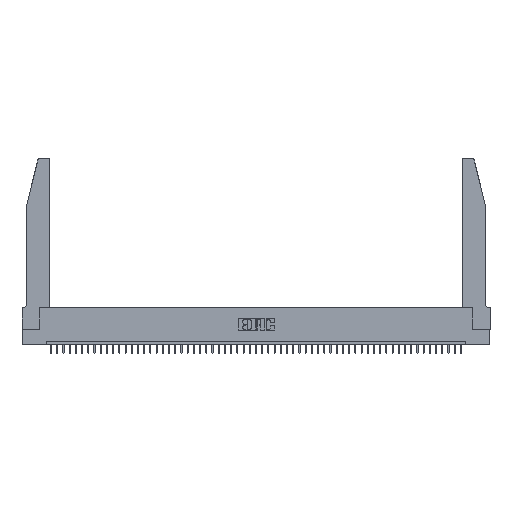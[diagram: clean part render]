
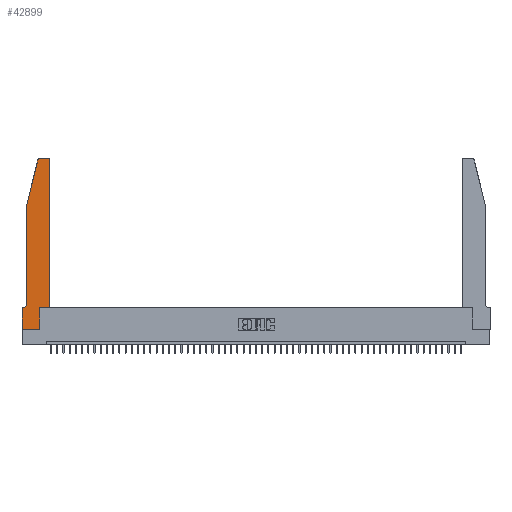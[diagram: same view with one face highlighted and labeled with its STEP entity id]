
A CAD part, top view. The second image highlights one B-rep face of the part: STEP entity #42899.
In plain terms, the highlighted planar face has unit normal (0, 0, 1).
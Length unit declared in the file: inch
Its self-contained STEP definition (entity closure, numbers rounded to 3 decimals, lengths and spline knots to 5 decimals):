
#58 = CARTESIAN_POINT ( 'NONE',  ( 0., 0., 0.37 ) ) ;
#282 = CARTESIAN_POINT ( 'NONE',  ( 0.0755, 2., 0.37 ) ) ;
#797 = LINE ( 'NONE', #282, #17827 ) ;
#1139 = VERTEX_POINT ( 'NONE', #1203 ) ;
#1203 = CARTESIAN_POINT ( 'NONE',  ( 0.4505, 2.72, 0.37 ) ) ;
#2063 = EDGE_CURVE ( 'NONE', #24006, #1139, #30928, .T. ) ;
#2872 = LINE ( 'NONE', #50670, #32849 ) ;
#2934 = CARTESIAN_POINT ( 'NONE',  ( 0.2865, 0.35, 0.37 ) ) ;
#3099 = CARTESIAN_POINT ( 'NONE',  ( 0.4505, 0.35, 0.37 ) ) ;
#3978 = LINE ( 'NONE', #7670, #49486 ) ;
#4060 = EDGE_CURVE ( 'NONE', #22851, #24006, #2872, .T. ) ;
#4466 = DIRECTION ( 'NONE',  ( 0., -1., 0. ) ) ;
#5199 = DIRECTION ( 'NONE',  ( 1., 0., 0. ) ) ;
#5670 = CIRCLE ( 'NONE', #44254, 0.03 ) ;
#5770 = CARTESIAN_POINT ( 'NONE',  ( 0., 0., 0.37 ) ) ;
#5868 = CARTESIAN_POINT ( 'NONE',  ( 0.25487, 2.72718, 0.37 ) ) ;
#6848 = LINE ( 'NONE', #15014, #40500 ) ;
#7275 = LINE ( 'NONE', #35645, #19015 ) ;
#7537 = CARTESIAN_POINT ( 'NONE',  ( 0.0055, 0.42, 0.37 ) ) ;
#7670 = CARTESIAN_POINT ( 'NONE',  ( 0., 0., 0.37 ) ) ;
#7699 = VERTEX_POINT ( 'NONE', #12435 ) ;
#7928 = DIRECTION ( 'NONE',  ( 0., -1., 0. ) ) ;
#8162 = ORIENTED_EDGE ( 'NONE', *, *, #10719, .T. ) ;
#8894 = CARTESIAN_POINT ( 'NONE',  ( 0.2865, 0., 0.37 ) ) ;
#8969 = CARTESIAN_POINT ( 'NONE',  ( 0.4205, 2.72, 0.37 ) ) ;
#9206 = LINE ( 'NONE', #15634, #21883 ) ;
#10719 = EDGE_CURVE ( 'NONE', #27267, #36600, #7275, .T. ) ;
#10942 = AXIS2_PLACEMENT_3D ( 'NONE', #7537, #26726, #31436 ) ;
#12435 = CARTESIAN_POINT ( 'NONE',  ( 0., 0.35, 0.37 ) ) ;
#12593 = CARTESIAN_POINT ( 'NONE',  ( 0.0755, 2., 0.37 ) ) ;
#12854 = VERTEX_POINT ( 'NONE', #8894 ) ;
#13060 = DIRECTION ( 'NONE',  ( 0., 0., 1. ) ) ;
#14085 = EDGE_CURVE ( 'NONE', #1139, #45337, #5670, .T. ) ;
#15014 = CARTESIAN_POINT ( 'NONE',  ( 0.2605, 2.75, 0.37 ) ) ;
#15447 = DIRECTION ( 'NONE',  ( -0.239, -0.971, 0. ) ) ;
#15573 = VERTEX_POINT ( 'NONE', #21575 ) ;
#15634 = CARTESIAN_POINT ( 'NONE',  ( 0.0755, 0.35, 0.37 ) ) ;
#16231 = CARTESIAN_POINT ( 'NONE',  ( 0.2865, 0.35, 0.37 ) ) ;
#17080 = EDGE_CURVE ( 'NONE', #33420, #46485, #31923, .T. ) ;
#17699 = EDGE_CURVE ( 'NONE', #46485, #7699, #9206, .T. ) ;
#17827 = VECTOR ( 'NONE', #4466, 39.37008 ) ;
#17942 = VERTEX_POINT ( 'NONE', #5770 ) ;
#19015 = VECTOR ( 'NONE', #15447, 39.37008 ) ;
#19821 = DIRECTION ( 'NONE',  ( -1., 0., 0. ) ) ;
#20423 = FACE_OUTER_BOUND ( 'NONE', #46951, .T. ) ;
#21575 = CARTESIAN_POINT ( 'NONE',  ( 0.284, 2.75, 0.37 ) ) ;
#21883 = VECTOR ( 'NONE', #19821, 39.37008 ) ;
#22851 = VERTEX_POINT ( 'NONE', #16231 ) ;
#22886 = VECTOR ( 'NONE', #35228, 39.37008 ) ;
#24006 = VERTEX_POINT ( 'NONE', #26316 ) ;
#25181 = CARTESIAN_POINT ( 'NONE',  ( 0.284, 2.72, 0.37 ) ) ;
#26316 = CARTESIAN_POINT ( 'NONE',  ( 0.4505, 0.35, 0.37 ) ) ;
#26726 = DIRECTION ( 'NONE',  ( 0., 0., -1. ) ) ;
#26772 = DIRECTION ( 'NONE',  ( 1., 0., 0. ) ) ;
#26847 = ORIENTED_EDGE ( 'NONE', *, *, #17080, .T. ) ;
#27267 = VERTEX_POINT ( 'NONE', #5868 ) ;
#27919 = DIRECTION ( 'NONE',  ( 0., 0., 1. ) ) ;
#30351 = DIRECTION ( 'NONE',  ( 0., 0., 1. ) ) ;
#30865 = EDGE_CURVE ( 'NONE', #15573, #27267, #43033, .T. ) ;
#30928 = LINE ( 'NONE', #3099, #36375 ) ;
#30949 = CARTESIAN_POINT ( 'NONE',  ( 0.0755, 0.42, 0.37 ) ) ;
#31335 = ORIENTED_EDGE ( 'NONE', *, *, #14085, .T. ) ;
#31436 = DIRECTION ( 'NONE',  ( -1., 0., 0. ) ) ;
#31923 = CIRCLE ( 'NONE', #10942, 0.07 ) ;
#32849 = VECTOR ( 'NONE', #26772, 39.37008 ) ;
#32941 = EDGE_CURVE ( 'NONE', #45337, #15573, #6848, .T. ) ;
#33420 = VERTEX_POINT ( 'NONE', #30949 ) ;
#33550 = LINE ( 'NONE', #58, #46952 ) ;
#35131 = DIRECTION ( 'NONE',  ( 0., 1., 0. ) ) ;
#35228 = DIRECTION ( 'NONE',  ( 0., 1., 0. ) ) ;
#35645 = CARTESIAN_POINT ( 'NONE',  ( 0.0755, 2., 0.37 ) ) ;
#36375 = VECTOR ( 'NONE', #35131, 39.37008 ) ;
#36442 = PLANE ( 'NONE',  #43756 ) ;
#36600 = VERTEX_POINT ( 'NONE', #12593 ) ;
#37291 = ORIENTED_EDGE ( 'NONE', *, *, #30865, .T. ) ;
#37612 = ORIENTED_EDGE ( 'NONE', *, *, #32941, .T. ) ;
#37977 = AXIS2_PLACEMENT_3D ( 'NONE', #25181, #30351, #5199 ) ;
#37980 = ORIENTED_EDGE ( 'NONE', *, *, #2063, .T. ) ;
#38198 = ORIENTED_EDGE ( 'NONE', *, *, #39402, .T. ) ;
#38375 = DIRECTION ( 'NONE',  ( -1., 0., 0. ) ) ;
#38918 = LINE ( 'NONE', #2934, #22886 ) ;
#39402 = EDGE_CURVE ( 'NONE', #7699, #17942, #3978, .T. ) ;
#39482 = EDGE_CURVE ( 'NONE', #17942, #12854, #33550, .T. ) ;
#40500 = VECTOR ( 'NONE', #38375, 39.37008 ) ;
#40999 = DIRECTION ( 'NONE',  ( 1., 0., 0. ) ) ;
#41942 = DIRECTION ( 'NONE',  ( 1., 0., 0. ) ) ;
#42143 = CARTESIAN_POINT ( 'NONE',  ( 0.0055, 0.35, 0.37 ) ) ;
#42899 = ADVANCED_FACE ( 'NONE', ( #20423 ), #36442, .T. ) ;
#43033 = CIRCLE ( 'NONE', #37977, 0.03 ) ;
#43756 = AXIS2_PLACEMENT_3D ( 'NONE', #48513, #13060, #49023 ) ;
#43960 = ORIENTED_EDGE ( 'NONE', *, *, #44112, .T. ) ;
#44076 = EDGE_CURVE ( 'NONE', #12854, #22851, #38918, .T. ) ;
#44112 = EDGE_CURVE ( 'NONE', #36600, #33420, #797, .T. ) ;
#44254 = AXIS2_PLACEMENT_3D ( 'NONE', #8969, #27919, #40999 ) ;
#45337 = VERTEX_POINT ( 'NONE', #48593 ) ;
#46485 = VERTEX_POINT ( 'NONE', #42143 ) ;
#46951 = EDGE_LOOP ( 'NONE', ( #37612, #37291, #8162, #43960, #26847, #50676, #38198, #51142, #49690, #51333, #37980, #31335 ) ) ;
#46952 = VECTOR ( 'NONE', #41942, 39.37008 ) ;
#48513 = CARTESIAN_POINT ( 'NONE',  ( 0., 0.35, 0.37 ) ) ;
#48593 = CARTESIAN_POINT ( 'NONE',  ( 0.4205, 2.75, 0.37 ) ) ;
#49023 = DIRECTION ( 'NONE',  ( 1., 0., 0. ) ) ;
#49486 = VECTOR ( 'NONE', #7928, 39.37008 ) ;
#49690 = ORIENTED_EDGE ( 'NONE', *, *, #44076, .T. ) ;
#50670 = CARTESIAN_POINT ( 'NONE',  ( 0.4505, 0.35, 0.37 ) ) ;
#50676 = ORIENTED_EDGE ( 'NONE', *, *, #17699, .T. ) ;
#51142 = ORIENTED_EDGE ( 'NONE', *, *, #39482, .T. ) ;
#51333 = ORIENTED_EDGE ( 'NONE', *, *, #4060, .T. ) ;
